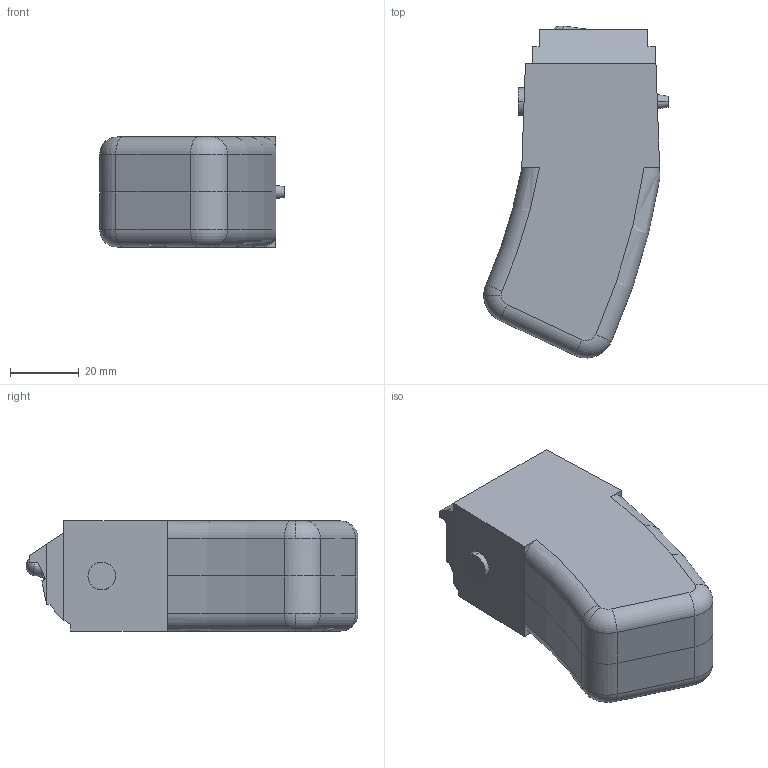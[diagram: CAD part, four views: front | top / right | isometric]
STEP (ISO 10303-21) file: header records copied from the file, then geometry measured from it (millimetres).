
FILE_DESCRIPTION (( 'STEP AP214' ), '1' );
FILE_NAME ('10rd_magazine.STEP', '2013-06-30T23:56:49', ( '' ), ( '' ), 'SwSTEP 2.0', 'SolidWorks 2013', '' );
FILE_SCHEMA (( 'AUTOMOTIVE_DESIGN' ));
Length unit declared in the file: millimetre
Products named in the file (8): 22LR-Case; left_small; right_small; 10rd_magazine; roller; follower; 22LR; 22LR-Bullet
Assembly tree (16 placements, depth 3):
  10rd_magazine
    right_small
    left_small
    22LR  x10
      22LR-Case
      22LR-Bullet
    follower
    roller
Bounding box: 53.52 x 96.36 x 32 mm (x, y, z)
Volume: 75233.6 mm3; surface area: 43460.1 mm2
Topology: 24 solids, 24 shells, 441 faces, 1051 edges, 665 vertices
Faces by surface type: plane 202, cylinder 169, torus 61, sphere 4, bspline 3, cone 2
Entity records: 9264 total; most frequent: CARTESIAN_POINT 1856, DIRECTION 1537, ORIENTED_EDGE 1478, EDGE_CURVE 739, AXIS2_PLACEMENT_3D 544, VERTEX_POINT 476, VECTOR 449, LINE 449
